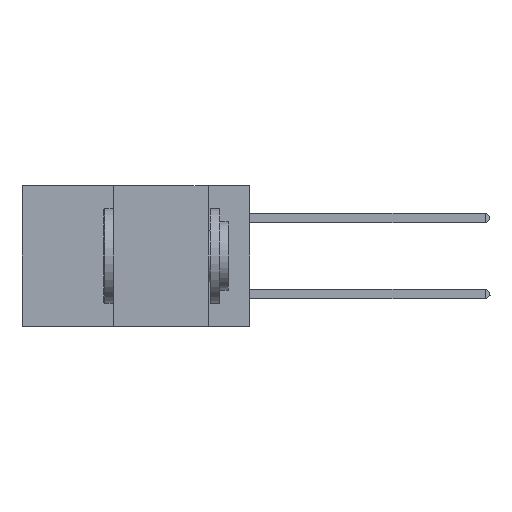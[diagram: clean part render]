
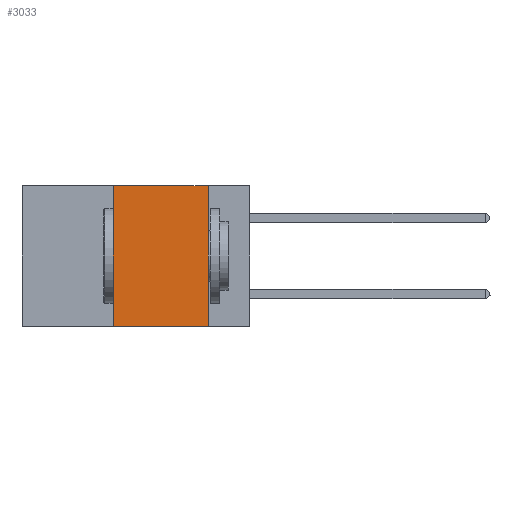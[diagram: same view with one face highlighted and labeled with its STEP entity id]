
A CAD part, left-side view. The second image highlights one B-rep face of the part: STEP entity #3033.
In plain terms, the highlighted planar face has unit normal (-1, 0, 0).
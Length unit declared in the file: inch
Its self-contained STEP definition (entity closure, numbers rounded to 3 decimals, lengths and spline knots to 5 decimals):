
#85 = LINE ( 'NONE', #18527, #10767 ) ;
#492 = EDGE_CURVE ( 'NONE', #16774, #22269, #15410, .T. ) ;
#872 = DIRECTION ( 'NONE',  ( 0., -1., 0. ) ) ;
#1001 = VERTEX_POINT ( 'NONE', #19039 ) ;
#1039 = ORIENTED_EDGE ( 'NONE', *, *, #5676, .F. ) ;
#1776 = VECTOR ( 'NONE', #14389, 39.37008 ) ;
#3033 = ADVANCED_FACE ( 'NONE', ( #8173 ), #8405, .F. ) ;
#4096 = ORIENTED_EDGE ( 'NONE', *, *, #492, .F. ) ;
#5604 = LINE ( 'NONE', #17748, #9422 ) ;
#5676 = EDGE_CURVE ( 'NONE', #22269, #22393, #15989, .T. ) ;
#6166 = DIRECTION ( 'NONE',  ( 0., 0., 1. ) ) ;
#6442 = CARTESIAN_POINT ( 'NONE',  ( 0., 0.6, 0. ) ) ;
#7920 = EDGE_CURVE ( 'NONE', #22393, #1001, #85, .T. ) ;
#8173 = FACE_OUTER_BOUND ( 'NONE', #17425, .T. ) ;
#8340 = ORIENTED_EDGE ( 'NONE', *, *, #14864, .T. ) ;
#8405 = PLANE ( 'NONE',  #16226 ) ;
#9422 = VECTOR ( 'NONE', #872, 39.37008 ) ;
#9523 = ORIENTED_EDGE ( 'NONE', *, *, #7920, .F. ) ;
#9695 = DIRECTION ( 'NONE',  ( 0., 0., -1. ) ) ;
#10767 = VECTOR ( 'NONE', #9695, 39.37008 ) ;
#10801 = CARTESIAN_POINT ( 'NONE',  ( 0., 0.36, -0.37 ) ) ;
#12248 = DIRECTION ( 'NONE',  ( 0., 0., -1. ) ) ;
#12369 = CARTESIAN_POINT ( 'NONE',  ( 0., 0.11, 0. ) ) ;
#12915 = CARTESIAN_POINT ( 'NONE',  ( 0., 0.36, 0. ) ) ;
#14311 = CARTESIAN_POINT ( 'NONE',  ( 0., 0.6, 0. ) ) ;
#14389 = DIRECTION ( 'NONE',  ( 0., -1., 0. ) ) ;
#14864 = EDGE_CURVE ( 'NONE', #16774, #1001, #5604, .T. ) ;
#15410 = LINE ( 'NONE', #21892, #15946 ) ;
#15946 = VECTOR ( 'NONE', #6166, 39.37008 ) ;
#15989 = LINE ( 'NONE', #14311, #1776 ) ;
#16226 = AXIS2_PLACEMENT_3D ( 'NONE', #6442, #21067, #12248 ) ;
#16774 = VERTEX_POINT ( 'NONE', #10801 ) ;
#17425 = EDGE_LOOP ( 'NONE', ( #9523, #1039, #4096, #8340 ) ) ;
#17748 = CARTESIAN_POINT ( 'NONE',  ( 0., 0.6, -0.37 ) ) ;
#18527 = CARTESIAN_POINT ( 'NONE',  ( 0., 0.11, 0. ) ) ;
#19039 = CARTESIAN_POINT ( 'NONE',  ( 0., 0.11, -0.37 ) ) ;
#21067 = DIRECTION ( 'NONE',  ( 1., 0., 0. ) ) ;
#21892 = CARTESIAN_POINT ( 'NONE',  ( 0., 0.36, 0. ) ) ;
#22269 = VERTEX_POINT ( 'NONE', #12915 ) ;
#22393 = VERTEX_POINT ( 'NONE', #12369 ) ;
